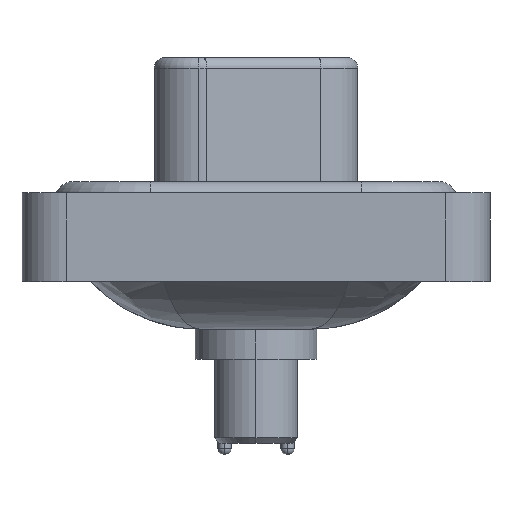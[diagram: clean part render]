
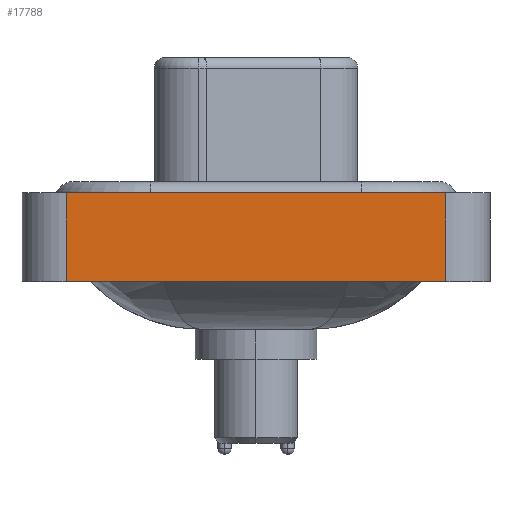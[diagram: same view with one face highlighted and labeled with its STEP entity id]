
A CAD part, left-side view. The second image highlights one B-rep face of the part: STEP entity #17788.
In plain terms, the highlighted planar face has unit normal (-1, 0, 0).
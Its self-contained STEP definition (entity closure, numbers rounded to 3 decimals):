
#1423 = DIRECTION ( 'NONE',  ( 0., 0., 1. ) ) ;
#1554 = ORIENTED_EDGE ( 'NONE', *, *, #16570, .T. ) ;
#2074 = AXIS2_PLACEMENT_3D ( 'NONE', #21451, #16679, #12992 ) ;
#3189 = LINE ( 'NONE', #21948, #8398 ) ;
#3482 = VECTOR ( 'NONE', #4918, 1000. ) ;
#4126 = VECTOR ( 'NONE', #12163, 1000. ) ;
#4866 = EDGE_CURVE ( 'NONE', #7727, #10843, #5960, .T. ) ;
#4918 = DIRECTION ( 'NONE',  ( 0., -1., 0. ) ) ;
#5418 = CARTESIAN_POINT ( 'NONE',  ( -7.35, -8.55, -3.6 ) ) ;
#5960 = LINE ( 'NONE', #12706, #17065 ) ;
#6265 = CARTESIAN_POINT ( 'NONE',  ( -7.35, 8.55, -3.6 ) ) ;
#7727 = VERTEX_POINT ( 'NONE', #14688 ) ;
#7815 = VERTEX_POINT ( 'NONE', #6265 ) ;
#8398 = VECTOR ( 'NONE', #1423, 1000. ) ;
#10585 = EDGE_CURVE ( 'NONE', #15625, #10843, #13124, .T. ) ;
#10750 = CARTESIAN_POINT ( 'NONE',  ( -7.35, -8.55, 0.4 ) ) ;
#10843 = VERTEX_POINT ( 'NONE', #10750 ) ;
#11521 = ORIENTED_EDGE ( 'NONE', *, *, #15212, .F. ) ;
#12015 = ORIENTED_EDGE ( 'NONE', *, *, #10585, .F. ) ;
#12163 = DIRECTION ( 'NONE',  ( 0., -1., 0. ) ) ;
#12706 = CARTESIAN_POINT ( 'NONE',  ( -7.35, -8.55, -3.6 ) ) ;
#12992 = DIRECTION ( 'NONE',  ( 0., 0., 1. ) ) ;
#13124 = LINE ( 'NONE', #19924, #3482 ) ;
#14666 = PLANE ( 'NONE',  #2074 ) ;
#14688 = CARTESIAN_POINT ( 'NONE',  ( -7.35, -8.55, -3.6 ) ) ;
#15212 = EDGE_CURVE ( 'NONE', #7815, #15625, #3189, .T. ) ;
#15625 = VERTEX_POINT ( 'NONE', #18283 ) ;
#16570 = EDGE_CURVE ( 'NONE', #7815, #7727, #20633, .T. ) ;
#16679 = DIRECTION ( 'NONE',  ( -1., 0., 0. ) ) ;
#16864 = EDGE_LOOP ( 'NONE', ( #19627, #12015, #11521, #1554 ) ) ;
#17065 = VECTOR ( 'NONE', #19161, 1000. ) ;
#17788 = ADVANCED_FACE ( 'NONE', ( #19679 ), #14666, .T. ) ;
#18283 = CARTESIAN_POINT ( 'NONE',  ( -7.35, 8.55, 0.4 ) ) ;
#19161 = DIRECTION ( 'NONE',  ( 0., 0., 1. ) ) ;
#19627 = ORIENTED_EDGE ( 'NONE', *, *, #4866, .T. ) ;
#19679 = FACE_OUTER_BOUND ( 'NONE', #16864, .T. ) ;
#19924 = CARTESIAN_POINT ( 'NONE',  ( -7.35, -8.55, 0.4 ) ) ;
#20633 = LINE ( 'NONE', #5418, #4126 ) ;
#21451 = CARTESIAN_POINT ( 'NONE',  ( -7.35, -8.55, -3.6 ) ) ;
#21948 = CARTESIAN_POINT ( 'NONE',  ( -7.35, 8.55, -3.6 ) ) ;
